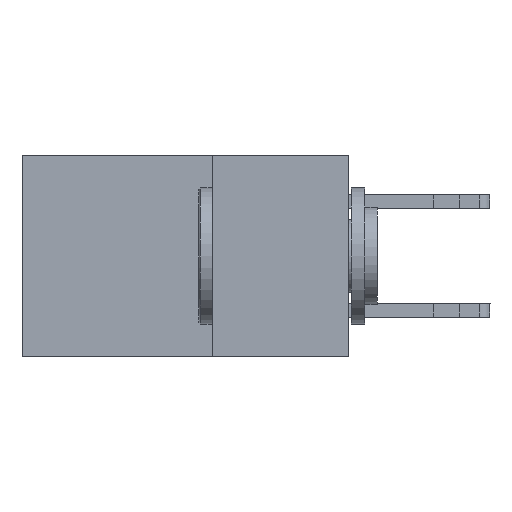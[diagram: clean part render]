
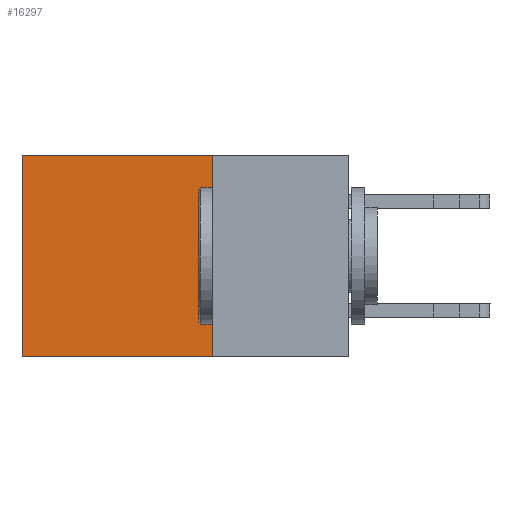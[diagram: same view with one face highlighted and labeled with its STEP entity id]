
A CAD part, left-side view. The second image highlights one B-rep face of the part: STEP entity #16297.
In plain terms, the highlighted planar face has unit normal (-1, 0, 0).
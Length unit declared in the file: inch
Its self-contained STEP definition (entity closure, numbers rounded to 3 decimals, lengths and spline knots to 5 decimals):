
#939 = VECTOR ( 'NONE', #11435, 39.37008 ) ;
#1209 = CARTESIAN_POINT ( 'NONE',  ( 0.2615, 0.25, -0.37 ) ) ;
#1253 = EDGE_CURVE ( 'NONE', #4873, #10989, #4211, .T. ) ;
#1924 = LINE ( 'NONE', #8046, #5355 ) ;
#1978 = EDGE_CURVE ( 'NONE', #13901, #6862, #14792, .T. ) ;
#2031 = ORIENTED_EDGE ( 'NONE', *, *, #1253, .F. ) ;
#2778 = ORIENTED_EDGE ( 'NONE', *, *, #3596, .F. ) ;
#3101 = CARTESIAN_POINT ( 'NONE',  ( 0.2615, 0.6, -0.37 ) ) ;
#3489 = VECTOR ( 'NONE', #9566, 39.37008 ) ;
#3596 = EDGE_CURVE ( 'NONE', #10989, #6862, #4815, .T. ) ;
#3625 = ORIENTED_EDGE ( 'NONE', *, *, #1978, .T. ) ;
#4170 = PLANE ( 'NONE',  #6724 ) ;
#4211 = LINE ( 'NONE', #6792, #15904 ) ;
#4815 = LINE ( 'NONE', #11530, #939 ) ;
#4873 = VERTEX_POINT ( 'NONE', #16692 ) ;
#5355 = VECTOR ( 'NONE', #9450, 39.37008 ) ;
#5619 = DIRECTION ( 'NONE',  ( 1., 0., 0. ) ) ;
#6495 = EDGE_CURVE ( 'NONE', #4873, #13901, #1924, .T. ) ;
#6724 = AXIS2_PLACEMENT_3D ( 'NONE', #1209, #5619, #15455 ) ;
#6792 = CARTESIAN_POINT ( 'NONE',  ( 0.2615, 0.25, -0.37 ) ) ;
#6862 = VERTEX_POINT ( 'NONE', #3101 ) ;
#7584 = CARTESIAN_POINT ( 'NONE',  ( 0.2615, 0.25, -0.37 ) ) ;
#8046 = CARTESIAN_POINT ( 'NONE',  ( 0.2615, 0.25, 0. ) ) ;
#9450 = DIRECTION ( 'NONE',  ( 0., 1., 0. ) ) ;
#9566 = DIRECTION ( 'NONE',  ( 0., 0., -1. ) ) ;
#10989 = VERTEX_POINT ( 'NONE', #7584 ) ;
#11435 = DIRECTION ( 'NONE',  ( 0., 1., 0. ) ) ;
#11530 = CARTESIAN_POINT ( 'NONE',  ( 0.2615, 0.25, -0.37 ) ) ;
#12099 = CARTESIAN_POINT ( 'NONE',  ( 0.2615, 0.6, 0. ) ) ;
#13121 = EDGE_LOOP ( 'NONE', ( #3625, #2778, #2031, #17643 ) ) ;
#13901 = VERTEX_POINT ( 'NONE', #12099 ) ;
#14792 = LINE ( 'NONE', #17280, #3489 ) ;
#15455 = DIRECTION ( 'NONE',  ( 0., 0., -1. ) ) ;
#15904 = VECTOR ( 'NONE', #18032, 39.37008 ) ;
#16297 = ADVANCED_FACE ( 'NONE', ( #17648 ), #4170, .F. ) ;
#16692 = CARTESIAN_POINT ( 'NONE',  ( 0.2615, 0.25, 0. ) ) ;
#17280 = CARTESIAN_POINT ( 'NONE',  ( 0.2615, 0.6, -0.37 ) ) ;
#17643 = ORIENTED_EDGE ( 'NONE', *, *, #6495, .T. ) ;
#17648 = FACE_OUTER_BOUND ( 'NONE', #13121, .T. ) ;
#18032 = DIRECTION ( 'NONE',  ( 0., 0., -1. ) ) ;
